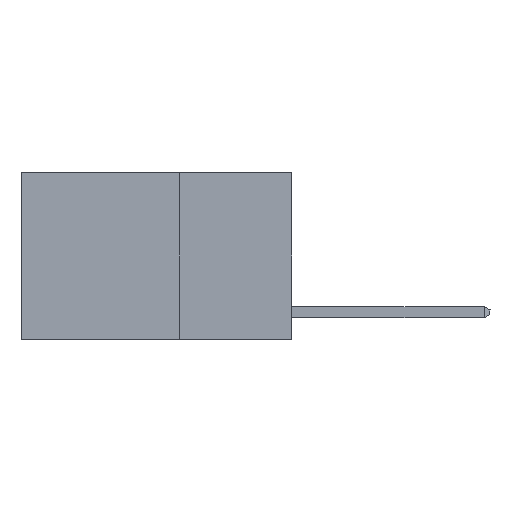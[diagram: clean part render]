
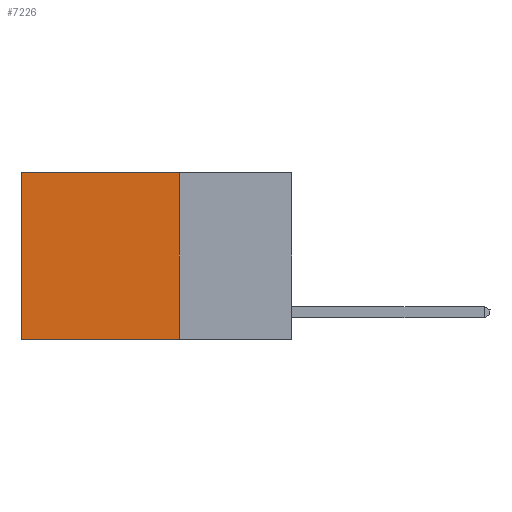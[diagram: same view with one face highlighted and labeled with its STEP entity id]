
A CAD part, left-side view. The second image highlights one B-rep face of the part: STEP entity #7226.
In plain terms, the highlighted planar face has unit normal (-1, 0, 0).
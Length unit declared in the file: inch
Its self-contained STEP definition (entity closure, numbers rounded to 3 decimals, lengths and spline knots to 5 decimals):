
#504 = CARTESIAN_POINT ( 'NONE',  ( 0.2625, 0.25, 0. ) ) ;
#996 = VECTOR ( 'NONE', #5519, 39.37008 ) ;
#1502 = EDGE_CURVE ( 'NONE', #20147, #11832, #11354, .T. ) ;
#1930 = VECTOR ( 'NONE', #2246, 39.37008 ) ;
#2246 = DIRECTION ( 'NONE',  ( 0., 1., 0. ) ) ;
#2630 = DIRECTION ( 'NONE',  ( 0., 0., -1. ) ) ;
#2867 = FACE_OUTER_BOUND ( 'NONE', #23561, .T. ) ;
#3032 = VERTEX_POINT ( 'NONE', #20345 ) ;
#3108 = CARTESIAN_POINT ( 'NONE',  ( 0.2625, 0.25, 0. ) ) ;
#4318 = CARTESIAN_POINT ( 'NONE',  ( 0.2625, 0.25, -0.37 ) ) ;
#4415 = VERTEX_POINT ( 'NONE', #7618 ) ;
#4800 = DIRECTION ( 'NONE',  ( 0., 1., 0. ) ) ;
#5519 = DIRECTION ( 'NONE',  ( 0., 0., -1. ) ) ;
#7226 = ADVANCED_FACE ( 'NONE', ( #2867 ), #13185, .F. ) ;
#7242 = EDGE_CURVE ( 'NONE', #11832, #4415, #7940, .T. ) ;
#7618 = CARTESIAN_POINT ( 'NONE',  ( 0.2625, 0.6, -0.37 ) ) ;
#7940 = LINE ( 'NONE', #17088, #12185 ) ;
#8134 = ORIENTED_EDGE ( 'NONE', *, *, #1502, .T. ) ;
#8752 = LINE ( 'NONE', #15803, #996 ) ;
#11212 = DIRECTION ( 'NONE',  ( 0., 0., -1. ) ) ;
#11354 = LINE ( 'NONE', #504, #16029 ) ;
#11713 = ORIENTED_EDGE ( 'NONE', *, *, #7242, .T. ) ;
#11832 = VERTEX_POINT ( 'NONE', #14851 ) ;
#12185 = VECTOR ( 'NONE', #11212, 39.37008 ) ;
#13185 = PLANE ( 'NONE',  #14913 ) ;
#13199 = LINE ( 'NONE', #4318, #1930 ) ;
#13775 = EDGE_CURVE ( 'NONE', #20147, #3032, #8752, .T. ) ;
#14851 = CARTESIAN_POINT ( 'NONE',  ( 0.2625, 0.6, 0. ) ) ;
#14913 = AXIS2_PLACEMENT_3D ( 'NONE', #24729, #15152, #2630 ) ;
#15152 = DIRECTION ( 'NONE',  ( 1., 0., 0. ) ) ;
#15625 = EDGE_CURVE ( 'NONE', #3032, #4415, #13199, .T. ) ;
#15803 = CARTESIAN_POINT ( 'NONE',  ( 0.2625, 0.25, 0. ) ) ;
#16029 = VECTOR ( 'NONE', #4800, 39.37008 ) ;
#17088 = CARTESIAN_POINT ( 'NONE',  ( 0.2625, 0.6, 0. ) ) ;
#20147 = VERTEX_POINT ( 'NONE', #3108 ) ;
#20345 = CARTESIAN_POINT ( 'NONE',  ( 0.2625, 0.25, -0.37 ) ) ;
#22103 = ORIENTED_EDGE ( 'NONE', *, *, #15625, .F. ) ;
#23329 = ORIENTED_EDGE ( 'NONE', *, *, #13775, .F. ) ;
#23561 = EDGE_LOOP ( 'NONE', ( #11713, #22103, #23329, #8134 ) ) ;
#24729 = CARTESIAN_POINT ( 'NONE',  ( 0.2625, 0.25, 0. ) ) ;
